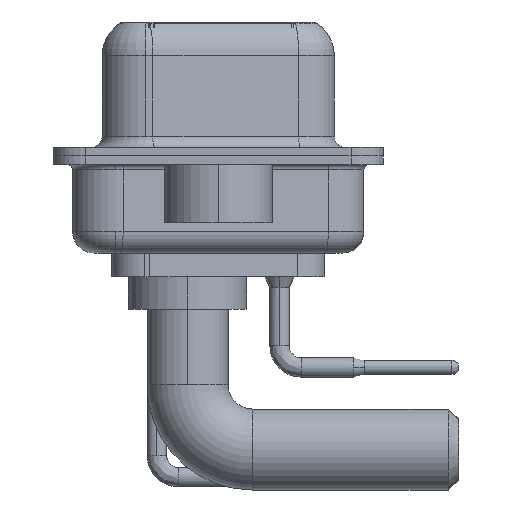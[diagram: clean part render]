
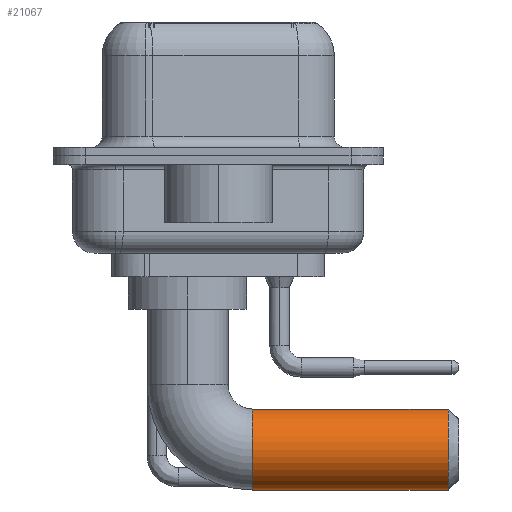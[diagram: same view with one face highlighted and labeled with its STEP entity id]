
A CAD part, left-side view. The second image highlights one B-rep face of the part: STEP entity #21067.
In plain terms, the highlighted cylindrical face has radius 1.875 mm (diameter 3.75 mm), a partial arc.
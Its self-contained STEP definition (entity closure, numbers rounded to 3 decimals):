
#259 = VERTEX_POINT ( 'NONE', #13243 ) ;
#420 = VERTEX_POINT ( 'NONE', #1889 ) ;
#472 = DIRECTION ( 'NONE',  ( 0., -1., 0. ) ) ;
#769 = CIRCLE ( 'NONE', #4593, 1.875 ) ;
#1664 = VECTOR ( 'NONE', #472, 1000. ) ;
#1889 = CARTESIAN_POINT ( 'NONE',  ( 0., -3., -4.625 ) ) ;
#2448 = ORIENTED_EDGE ( 'NONE', *, *, #31033, .F. ) ;
#4572 = LINE ( 'NONE', #28447, #16351 ) ;
#4593 = AXIS2_PLACEMENT_3D ( 'NONE', #8032, #17986, #10583 ) ;
#5458 = DIRECTION ( 'NONE',  ( 0., 0., -1. ) ) ;
#5629 = FACE_OUTER_BOUND ( 'NONE', #15706, .T. ) ;
#6908 = CARTESIAN_POINT ( 'NONE',  ( 0., -12.07, -4.625 ) ) ;
#7177 = EDGE_CURVE ( 'NONE', #420, #259, #769, .T. ) ;
#7374 = CARTESIAN_POINT ( 'NONE',  ( 0., -12.07, -8.375 ) ) ;
#8032 = CARTESIAN_POINT ( 'NONE',  ( 0., -3., -6.5 ) ) ;
#8218 = VERTEX_POINT ( 'NONE', #6908 ) ;
#8352 = LINE ( 'NONE', #32231, #1664 ) ;
#8399 = AXIS2_PLACEMENT_3D ( 'NONE', #18518, #23483, #5458 ) ;
#10583 = DIRECTION ( 'NONE',  ( -1., 0., 0. ) ) ;
#12303 = DIRECTION ( 'NONE',  ( 0., -1., 0. ) ) ;
#13009 = CYLINDRICAL_SURFACE ( 'NONE', #8399, 1.875 ) ;
#13243 = CARTESIAN_POINT ( 'NONE',  ( 0., -3., -8.375 ) ) ;
#15706 = EDGE_LOOP ( 'NONE', ( #2448, #21301, #21907, #33858 ) ) ;
#16351 = VECTOR ( 'NONE', #12303, 1000. ) ;
#16740 = CIRCLE ( 'NONE', #30998, 1.875 ) ;
#17986 = DIRECTION ( 'NONE',  ( 0., -1., 0. ) ) ;
#18116 = DIRECTION ( 'NONE',  ( 0., 0., -1. ) ) ;
#18518 = CARTESIAN_POINT ( 'NONE',  ( 0., -3., -6.5 ) ) ;
#20846 = VERTEX_POINT ( 'NONE', #7374 ) ;
#21067 = ADVANCED_FACE ( 'NONE', ( #5629 ), #13009, .T. ) ;
#21301 = ORIENTED_EDGE ( 'NONE', *, *, #7177, .T. ) ;
#21907 = ORIENTED_EDGE ( 'NONE', *, *, #29090, .T. ) ;
#23483 = DIRECTION ( 'NONE',  ( 0., -1., 0. ) ) ;
#24076 = EDGE_CURVE ( 'NONE', #20846, #8218, #16740, .T. ) ;
#28447 = CARTESIAN_POINT ( 'NONE',  ( 0., -3., -8.375 ) ) ;
#29090 = EDGE_CURVE ( 'NONE', #259, #20846, #4572, .T. ) ;
#29576 = CARTESIAN_POINT ( 'NONE',  ( 0., -12.07, -6.5 ) ) ;
#30998 = AXIS2_PLACEMENT_3D ( 'NONE', #29576, #33751, #18116 ) ;
#31033 = EDGE_CURVE ( 'NONE', #420, #8218, #8352, .T. ) ;
#32231 = CARTESIAN_POINT ( 'NONE',  ( 0., -3., -4.625 ) ) ;
#33751 = DIRECTION ( 'NONE',  ( 0., 1., 0. ) ) ;
#33858 = ORIENTED_EDGE ( 'NONE', *, *, #24076, .T. ) ;
